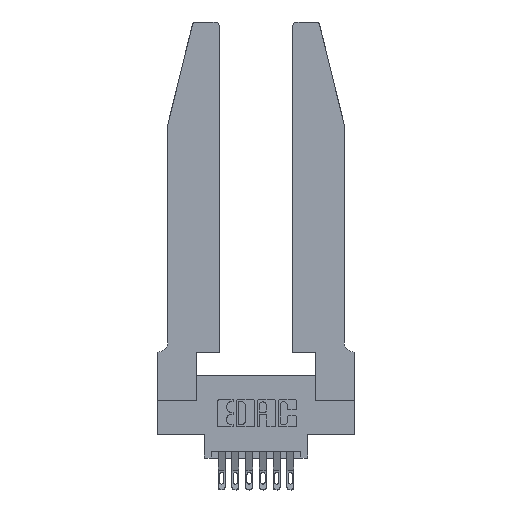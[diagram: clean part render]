
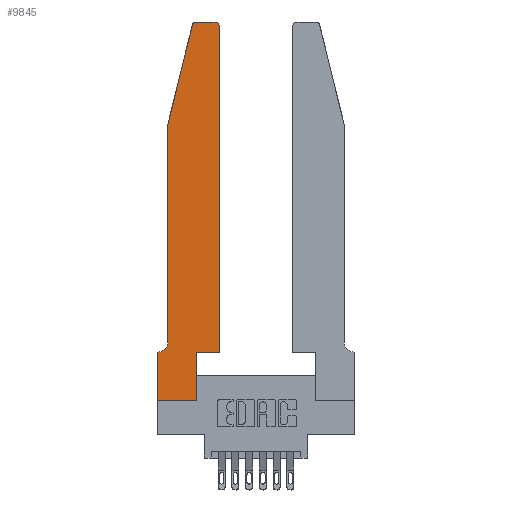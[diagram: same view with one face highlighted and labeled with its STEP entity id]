
A CAD part, top view. The second image highlights one B-rep face of the part: STEP entity #9845.
In plain terms, the highlighted planar face has unit normal (0, 0, 1).
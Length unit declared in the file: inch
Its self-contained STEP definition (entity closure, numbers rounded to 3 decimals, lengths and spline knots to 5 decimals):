
#67 = DIRECTION ( 'NONE',  ( 1., 0., 0. ) ) ;
#144 = LINE ( 'NONE', #12182, #6150 ) ;
#330 = LINE ( 'NONE', #3319, #12276 ) ;
#334 = DIRECTION ( 'NONE',  ( 0., -1., 0. ) ) ;
#487 = ORIENTED_EDGE ( 'NONE', *, *, #1568, .T. ) ;
#522 = VERTEX_POINT ( 'NONE', #11103 ) ;
#538 = ORIENTED_EDGE ( 'NONE', *, *, #3250, .T. ) ;
#655 = VECTOR ( 'NONE', #334, 39.37008 ) ;
#794 = ORIENTED_EDGE ( 'NONE', *, *, #7308, .T. ) ;
#823 = ORIENTED_EDGE ( 'NONE', *, *, #8379, .T. ) ;
#854 = ORIENTED_EDGE ( 'NONE', *, *, #8011, .T. ) ;
#904 = ORIENTED_EDGE ( 'NONE', *, *, #2452, .T. ) ;
#1093 = CARTESIAN_POINT ( 'NONE',  ( 0.2865, 0.35, 0.37 ) ) ;
#1147 = EDGE_CURVE ( 'NONE', #12915, #7874, #12423, .T. ) ;
#1275 = ORIENTED_EDGE ( 'NONE', *, *, #6754, .T. ) ;
#1380 = ORIENTED_EDGE ( 'NONE', *, *, #11781, .T. ) ;
#1523 = VERTEX_POINT ( 'NONE', #6867 ) ;
#1568 = EDGE_CURVE ( 'NONE', #2730, #1523, #10541, .T. ) ;
#1740 = AXIS2_PLACEMENT_3D ( 'NONE', #10120, #10931, #67 ) ;
#1782 = ORIENTED_EDGE ( 'NONE', *, *, #12318, .T. ) ;
#1865 = ORIENTED_EDGE ( 'NONE', *, *, #1147, .T. ) ;
#2069 = CARTESIAN_POINT ( 'NONE',  ( 0., 0., 0.37 ) ) ;
#2218 = AXIS2_PLACEMENT_3D ( 'NONE', #13318, #6716, #14398 ) ;
#2280 = VERTEX_POINT ( 'NONE', #7554 ) ;
#2452 = EDGE_CURVE ( 'NONE', #522, #4778, #13536, .T. ) ;
#2478 = DIRECTION ( 'NONE',  ( 0., -1., 0. ) ) ;
#2625 = LINE ( 'NONE', #7122, #14186 ) ;
#2727 = CARTESIAN_POINT ( 'NONE',  ( 0.4505, 0.35, 0.37 ) ) ;
#2730 = VERTEX_POINT ( 'NONE', #1093 ) ;
#2735 = LINE ( 'NONE', #4326, #8889 ) ;
#3250 = EDGE_CURVE ( 'NONE', #7874, #9637, #9820, .T. ) ;
#3319 = CARTESIAN_POINT ( 'NONE',  ( 0.2865, 0.35, 0.37 ) ) ;
#3449 = PLANE ( 'NONE',  #8469 ) ;
#3488 = ORIENTED_EDGE ( 'NONE', *, *, #3887, .T. ) ;
#3887 = EDGE_CURVE ( 'NONE', #2280, #12915, #5704, .T. ) ;
#3939 = VERTEX_POINT ( 'NONE', #10430 ) ;
#4021 = CARTESIAN_POINT ( 'NONE',  ( 0.0055, 0.35, 0.37 ) ) ;
#4027 = AXIS2_PLACEMENT_3D ( 'NONE', #12300, #5585, #13348 ) ;
#4326 = CARTESIAN_POINT ( 'NONE',  ( 0.0755, 0.35, 0.37 ) ) ;
#4398 = CARTESIAN_POINT ( 'NONE',  ( 0.284, 2.75, 0.37 ) ) ;
#4466 = DIRECTION ( 'NONE',  ( 0., 1., 0. ) ) ;
#4595 = DIRECTION ( 'NONE',  ( 0., 0., 1. ) ) ;
#4778 = VERTEX_POINT ( 'NONE', #7699 ) ;
#4788 = DIRECTION ( 'NONE',  ( -0.239, -0.971, 0. ) ) ;
#4863 = VECTOR ( 'NONE', #12024, 39.37008 ) ;
#5080 = CARTESIAN_POINT ( 'NONE',  ( 0.0755, 0.42, 0.37 ) ) ;
#5137 = VERTEX_POINT ( 'NONE', #5080 ) ;
#5290 = CARTESIAN_POINT ( 'NONE',  ( 0.25487, 2.72718, 0.37 ) ) ;
#5585 = DIRECTION ( 'NONE',  ( 0., 0., 1. ) ) ;
#5704 = LINE ( 'NONE', #12566, #8422 ) ;
#6017 = FACE_OUTER_BOUND ( 'NONE', #13845, .T. ) ;
#6079 = ORIENTED_EDGE ( 'NONE', *, *, #9776, .T. ) ;
#6150 = VECTOR ( 'NONE', #6565, 39.37008 ) ;
#6565 = DIRECTION ( 'NONE',  ( 0., 1., 0. ) ) ;
#6688 = CIRCLE ( 'NONE', #4027, 0.03 ) ;
#6716 = DIRECTION ( 'NONE',  ( 0., 0., -1. ) ) ;
#6754 = EDGE_CURVE ( 'NONE', #3939, #2730, #330, .T. ) ;
#6823 = VERTEX_POINT ( 'NONE', #8062 ) ;
#6867 = CARTESIAN_POINT ( 'NONE',  ( 0.4505, 0.35, 0.37 ) ) ;
#7036 = DIRECTION ( 'NONE',  ( -1., 0., 0. ) ) ;
#7122 = CARTESIAN_POINT ( 'NONE',  ( 0.0755, 2., 0.37 ) ) ;
#7130 = CIRCLE ( 'NONE', #2218, 0.07 ) ;
#7308 = EDGE_CURVE ( 'NONE', #1523, #6823, #144, .T. ) ;
#7430 = CARTESIAN_POINT ( 'NONE',  ( 0.0755, 2., 0.37 ) ) ;
#7436 = VECTOR ( 'NONE', #11288, 39.37008 ) ;
#7554 = CARTESIAN_POINT ( 'NONE',  ( 0.4205, 2.75, 0.37 ) ) ;
#7699 = CARTESIAN_POINT ( 'NONE',  ( 0., 0., 0.37 ) ) ;
#7874 = VERTEX_POINT ( 'NONE', #5290 ) ;
#7967 = CARTESIAN_POINT ( 'NONE',  ( 0., 0., 0.37 ) ) ;
#8011 = EDGE_CURVE ( 'NONE', #6823, #2280, #6688, .T. ) ;
#8062 = CARTESIAN_POINT ( 'NONE',  ( 0.4505, 2.72, 0.37 ) ) ;
#8379 = EDGE_CURVE ( 'NONE', #9637, #5137, #2625, .T. ) ;
#8422 = VECTOR ( 'NONE', #7036, 39.37008 ) ;
#8469 = AXIS2_PLACEMENT_3D ( 'NONE', #13456, #4595, #12454 ) ;
#8889 = VECTOR ( 'NONE', #12207, 39.37008 ) ;
#9637 = VERTEX_POINT ( 'NONE', #7430 ) ;
#9776 = EDGE_CURVE ( 'NONE', #5137, #12707, #7130, .T. ) ;
#9820 = LINE ( 'NONE', #13678, #12710 ) ;
#9845 = ADVANCED_FACE ( 'NONE', ( #6017 ), #3449, .T. ) ;
#10120 = CARTESIAN_POINT ( 'NONE',  ( 0.284, 2.72, 0.37 ) ) ;
#10410 = LINE ( 'NONE', #7967, #7436 ) ;
#10430 = CARTESIAN_POINT ( 'NONE',  ( 0.2865, 0., 0.37 ) ) ;
#10541 = LINE ( 'NONE', #2727, #4863 ) ;
#10931 = DIRECTION ( 'NONE',  ( 0., 0., 1. ) ) ;
#11103 = CARTESIAN_POINT ( 'NONE',  ( 0., 0.35, 0.37 ) ) ;
#11288 = DIRECTION ( 'NONE',  ( 1., 0., 0. ) ) ;
#11781 = EDGE_CURVE ( 'NONE', #12707, #522, #2735, .T. ) ;
#12024 = DIRECTION ( 'NONE',  ( 1., 0., 0. ) ) ;
#12182 = CARTESIAN_POINT ( 'NONE',  ( 0.4505, 0.35, 0.37 ) ) ;
#12207 = DIRECTION ( 'NONE',  ( -1., 0., 0. ) ) ;
#12276 = VECTOR ( 'NONE', #4466, 39.37008 ) ;
#12300 = CARTESIAN_POINT ( 'NONE',  ( 0.4205, 2.72, 0.37 ) ) ;
#12318 = EDGE_CURVE ( 'NONE', #4778, #3939, #10410, .T. ) ;
#12423 = CIRCLE ( 'NONE', #1740, 0.03 ) ;
#12454 = DIRECTION ( 'NONE',  ( 1., 0., 0. ) ) ;
#12566 = CARTESIAN_POINT ( 'NONE',  ( 0.2605, 2.75, 0.37 ) ) ;
#12707 = VERTEX_POINT ( 'NONE', #4021 ) ;
#12710 = VECTOR ( 'NONE', #4788, 39.37008 ) ;
#12915 = VERTEX_POINT ( 'NONE', #4398 ) ;
#13318 = CARTESIAN_POINT ( 'NONE',  ( 0.0055, 0.42, 0.37 ) ) ;
#13348 = DIRECTION ( 'NONE',  ( 1., 0., 0. ) ) ;
#13456 = CARTESIAN_POINT ( 'NONE',  ( 0., 0.35, 0.37 ) ) ;
#13536 = LINE ( 'NONE', #2069, #655 ) ;
#13678 = CARTESIAN_POINT ( 'NONE',  ( 0.0755, 2., 0.37 ) ) ;
#13845 = EDGE_LOOP ( 'NONE', ( #3488, #1865, #538, #823, #6079, #1380, #904, #1782, #1275, #487, #794, #854 ) ) ;
#14186 = VECTOR ( 'NONE', #2478, 39.37008 ) ;
#14398 = DIRECTION ( 'NONE',  ( -1., 0., 0. ) ) ;
